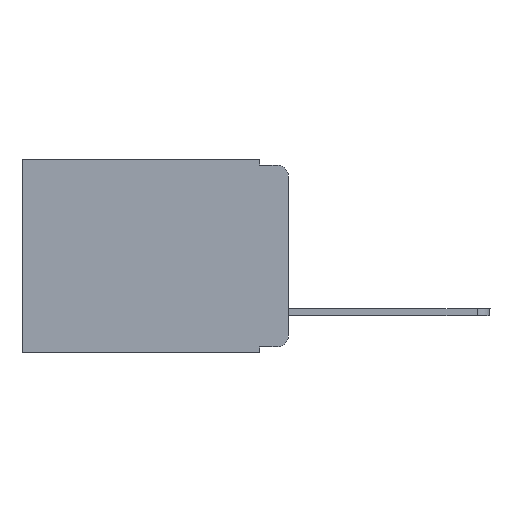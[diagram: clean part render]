
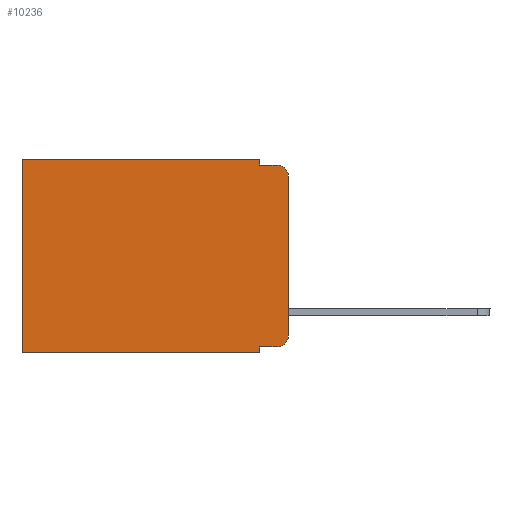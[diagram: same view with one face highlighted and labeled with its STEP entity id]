
A CAD part, left-side view. The second image highlights one B-rep face of the part: STEP entity #10236.
In plain terms, the highlighted planar face has unit normal (-1, 0, 0).
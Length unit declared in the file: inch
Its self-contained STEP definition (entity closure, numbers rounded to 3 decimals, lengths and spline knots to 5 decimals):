
#85 = DIRECTION ( 'NONE',  ( 0., 0., -1. ) ) ;
#230 = CARTESIAN_POINT ( 'NONE',  ( 0.298, 0., 0. ) ) ;
#295 = CARTESIAN_POINT ( 'NONE',  ( 0.298, 0.02, -0.333 ) ) ;
#299 = LINE ( 'NONE', #2951, #1087 ) ;
#322 = DIRECTION ( 'NONE',  ( 0., 0., -1. ) ) ;
#548 = LINE ( 'NONE', #2064, #7584 ) ;
#573 = DIRECTION ( 'NONE',  ( -1., 0., 0. ) ) ;
#586 = VECTOR ( 'NONE', #634, 39.37008 ) ;
#634 = DIRECTION ( 'NONE',  ( 0., -1., 0. ) ) ;
#701 = DIRECTION ( 'NONE',  ( 0., 0., -1. ) ) ;
#963 = LINE ( 'NONE', #8118, #3025 ) ;
#1087 = VECTOR ( 'NONE', #4879, 39.37008 ) ;
#1143 = DIRECTION ( 'NONE',  ( -1., 0., 0. ) ) ;
#1144 = VECTOR ( 'NONE', #701, 39.37008 ) ;
#1149 = EDGE_CURVE ( 'NONE', #1965, #7185, #3749, .T. ) ;
#1402 = EDGE_CURVE ( 'NONE', #7185, #1570, #10339, .T. ) ;
#1492 = AXIS2_PLACEMENT_3D ( 'NONE', #2017, #1143, #85 ) ;
#1545 = EDGE_CURVE ( 'NONE', #6710, #3064, #8669, .T. ) ;
#1546 = ORIENTED_EDGE ( 'NONE', *, *, #8448, .T. ) ;
#1570 = VERTEX_POINT ( 'NONE', #8787 ) ;
#1702 = CARTESIAN_POINT ( 'NONE',  ( 0.298, 0.473, 0. ) ) ;
#1853 = EDGE_CURVE ( 'NONE', #5225, #7161, #963, .T. ) ;
#1965 = VERTEX_POINT ( 'NONE', #3122 ) ;
#2017 = CARTESIAN_POINT ( 'NONE',  ( 0.298, 0.02, -0.03 ) ) ;
#2064 = CARTESIAN_POINT ( 'NONE',  ( 0.298, 0.051, 0. ) ) ;
#2105 = DIRECTION ( 'NONE',  ( 0., 1., 0. ) ) ;
#2361 = VERTEX_POINT ( 'NONE', #10245 ) ;
#2510 = CARTESIAN_POINT ( 'NONE',  ( 0.298, 0., -0.313 ) ) ;
#2572 = ORIENTED_EDGE ( 'NONE', *, *, #1545, .T. ) ;
#2829 = ORIENTED_EDGE ( 'NONE', *, *, #1853, .T. ) ;
#2899 = DIRECTION ( 'NONE',  ( 0., -1., 0. ) ) ;
#2951 = CARTESIAN_POINT ( 'NONE',  ( 0.298, 0., -0.343 ) ) ;
#3004 = DIRECTION ( 'NONE',  ( 1., 0., 0. ) ) ;
#3025 = VECTOR ( 'NONE', #2899, 39.37008 ) ;
#3028 = EDGE_LOOP ( 'NONE', ( #8639, #1546, #5511, #4529, #8211, #2572, #10279, #6516, #2829, #5012 ) ) ;
#3064 = VERTEX_POINT ( 'NONE', #6717 ) ;
#3122 = CARTESIAN_POINT ( 'NONE',  ( 0.298, 0.051, 0. ) ) ;
#3170 = CARTESIAN_POINT ( 'NONE',  ( 0.298, 0.051, -0.333 ) ) ;
#3749 = LINE ( 'NONE', #4509, #10038 ) ;
#3843 = AXIS2_PLACEMENT_3D ( 'NONE', #8311, #573, #322 ) ;
#3998 = DIRECTION ( 'NONE',  ( 0., 0., -1. ) ) ;
#4051 = VERTEX_POINT ( 'NONE', #2510 ) ;
#4068 = VERTEX_POINT ( 'NONE', #6860 ) ;
#4119 = VECTOR ( 'NONE', #2105, 39.37008 ) ;
#4509 = CARTESIAN_POINT ( 'NONE',  ( 0.298, 0.051, 0. ) ) ;
#4529 = ORIENTED_EDGE ( 'NONE', *, *, #1149, .F. ) ;
#4879 = DIRECTION ( 'NONE',  ( 0., 1., 0. ) ) ;
#4904 = LINE ( 'NONE', #8421, #5222 ) ;
#4992 = DIRECTION ( 'NONE',  ( 0., 0., -1. ) ) ;
#5012 = ORIENTED_EDGE ( 'NONE', *, *, #10947, .T. ) ;
#5222 = VECTOR ( 'NONE', #6687, 39.37008 ) ;
#5225 = VERTEX_POINT ( 'NONE', #3170 ) ;
#5511 = ORIENTED_EDGE ( 'NONE', *, *, #1402, .F. ) ;
#5697 = PLANE ( 'NONE',  #6664 ) ;
#6516 = ORIENTED_EDGE ( 'NONE', *, *, #10166, .F. ) ;
#6664 = AXIS2_PLACEMENT_3D ( 'NONE', #6722, #3004, #3998 ) ;
#6687 = DIRECTION ( 'NONE',  ( 0., 0., -1. ) ) ;
#6710 = VERTEX_POINT ( 'NONE', #7141 ) ;
#6717 = CARTESIAN_POINT ( 'NONE',  ( 0.298, 0.473, -0.343 ) ) ;
#6722 = CARTESIAN_POINT ( 'NONE',  ( 0.298, 0., 0. ) ) ;
#6860 = CARTESIAN_POINT ( 'NONE',  ( 0.298, 0., -0.03 ) ) ;
#6986 = CIRCLE ( 'NONE', #3843, 0.02 ) ;
#7141 = CARTESIAN_POINT ( 'NONE',  ( 0.298, 0.473, 0. ) ) ;
#7161 = VERTEX_POINT ( 'NONE', #295 ) ;
#7185 = VERTEX_POINT ( 'NONE', #8340 ) ;
#7584 = VECTOR ( 'NONE', #4992, 39.37008 ) ;
#7792 = CARTESIAN_POINT ( 'NONE',  ( 0.298, 0.051, -0.01 ) ) ;
#8118 = CARTESIAN_POINT ( 'NONE',  ( 0.298, 0.051, -0.333 ) ) ;
#8211 = ORIENTED_EDGE ( 'NONE', *, *, #8837, .T. ) ;
#8232 = EDGE_CURVE ( 'NONE', #4068, #4051, #4904, .T. ) ;
#8311 = CARTESIAN_POINT ( 'NONE',  ( 0.298, 0.02, -0.313 ) ) ;
#8340 = CARTESIAN_POINT ( 'NONE',  ( 0.298, 0.051, -0.01 ) ) ;
#8421 = CARTESIAN_POINT ( 'NONE',  ( 0.298, 0., 0. ) ) ;
#8448 = EDGE_CURVE ( 'NONE', #4068, #1570, #9096, .T. ) ;
#8639 = ORIENTED_EDGE ( 'NONE', *, *, #8232, .F. ) ;
#8669 = LINE ( 'NONE', #1702, #1144 ) ;
#8787 = CARTESIAN_POINT ( 'NONE',  ( 0.298, 0.02, -0.01 ) ) ;
#8837 = EDGE_CURVE ( 'NONE', #1965, #6710, #10056, .T. ) ;
#9096 = CIRCLE ( 'NONE', #1492, 0.02 ) ;
#9989 = DIRECTION ( 'NONE',  ( 0., 0., -1. ) ) ;
#10038 = VECTOR ( 'NONE', #9989, 39.37008 ) ;
#10056 = LINE ( 'NONE', #230, #4119 ) ;
#10163 = EDGE_CURVE ( 'NONE', #2361, #3064, #299, .T. ) ;
#10166 = EDGE_CURVE ( 'NONE', #5225, #2361, #548, .T. ) ;
#10236 = ADVANCED_FACE ( 'NONE', ( #10952 ), #5697, .F. ) ;
#10245 = CARTESIAN_POINT ( 'NONE',  ( 0.298, 0.051, -0.343 ) ) ;
#10279 = ORIENTED_EDGE ( 'NONE', *, *, #10163, .F. ) ;
#10339 = LINE ( 'NONE', #7792, #586 ) ;
#10947 = EDGE_CURVE ( 'NONE', #7161, #4051, #6986, .T. ) ;
#10952 = FACE_OUTER_BOUND ( 'NONE', #3028, .T. ) ;
